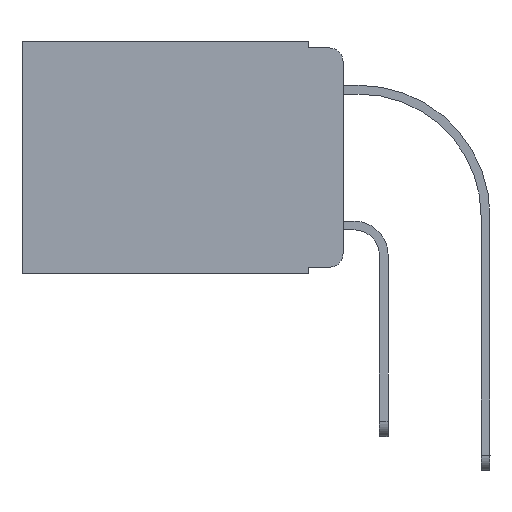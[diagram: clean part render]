
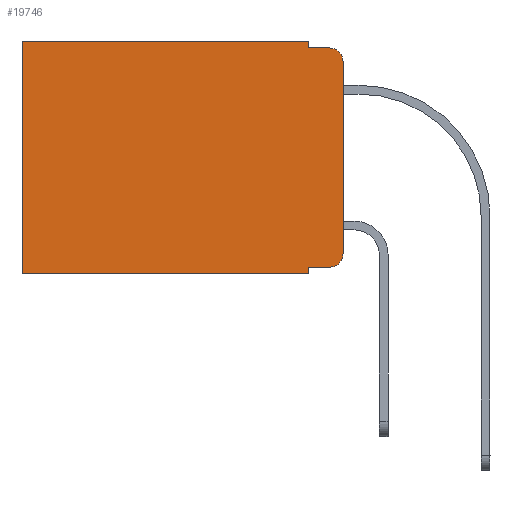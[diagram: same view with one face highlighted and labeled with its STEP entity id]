
A CAD part, left-side view. The second image highlights one B-rep face of the part: STEP entity #19746.
In plain terms, the highlighted planar face has unit normal (-1, 0, 0).
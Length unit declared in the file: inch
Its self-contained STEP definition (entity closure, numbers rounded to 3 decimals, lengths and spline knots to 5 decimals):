
#467 = LINE ( 'NONE', #2227, #14826 ) ;
#669 = CARTESIAN_POINT ( 'NONE',  ( 0.298, 0.051, -0.333 ) ) ;
#692 = DIRECTION ( 'NONE',  ( 0., -1., 0. ) ) ;
#709 = VECTOR ( 'NONE', #11517, 39.37008 ) ;
#900 = CARTESIAN_POINT ( 'NONE',  ( 0.298, 0.473, -0.343 ) ) ;
#1210 = VERTEX_POINT ( 'NONE', #2211 ) ;
#1388 = LINE ( 'NONE', #24292, #19934 ) ;
#1460 = DIRECTION ( 'NONE',  ( -1., 0., 0. ) ) ;
#1543 = CARTESIAN_POINT ( 'NONE',  ( 0.298, 0., 0. ) ) ;
#1808 = ORIENTED_EDGE ( 'NONE', *, *, #18998, .F. ) ;
#1936 = VERTEX_POINT ( 'NONE', #669 ) ;
#2211 = CARTESIAN_POINT ( 'NONE',  ( 0.298, 0.02, -0.01 ) ) ;
#2227 = CARTESIAN_POINT ( 'NONE',  ( 0.298, 0.473, 0. ) ) ;
#2429 = CARTESIAN_POINT ( 'NONE',  ( 0.298, 0.051, -0.01 ) ) ;
#2493 = VECTOR ( 'NONE', #692, 39.37008 ) ;
#3457 = VERTEX_POINT ( 'NONE', #18289 ) ;
#4311 = CIRCLE ( 'NONE', #19516, 0.02 ) ;
#4372 = EDGE_CURVE ( 'NONE', #1936, #24641, #10007, .T. ) ;
#4535 = ORIENTED_EDGE ( 'NONE', *, *, #16667, .F. ) ;
#4623 = ORIENTED_EDGE ( 'NONE', *, *, #20258, .T. ) ;
#4894 = VECTOR ( 'NONE', #12229, 39.37008 ) ;
#5232 = ORIENTED_EDGE ( 'NONE', *, *, #9940, .T. ) ;
#6278 = ORIENTED_EDGE ( 'NONE', *, *, #4372, .T. ) ;
#8195 = PLANE ( 'NONE',  #19969 ) ;
#8224 = CARTESIAN_POINT ( 'NONE',  ( 0.298, 0.051, 0. ) ) ;
#8313 = LINE ( 'NONE', #10929, #18620 ) ;
#8447 = DIRECTION ( 'NONE',  ( 1., 0., 0. ) ) ;
#8999 = VERTEX_POINT ( 'NONE', #2429 ) ;
#9044 = DIRECTION ( 'NONE',  ( 0., 0., -1. ) ) ;
#9327 = DIRECTION ( 'NONE',  ( 0., 1., 0. ) ) ;
#9650 = ORIENTED_EDGE ( 'NONE', *, *, #10064, .F. ) ;
#9698 = ORIENTED_EDGE ( 'NONE', *, *, #10687, .T. ) ;
#9940 = EDGE_CURVE ( 'NONE', #18014, #24470, #467, .T. ) ;
#10007 = LINE ( 'NONE', #19175, #709 ) ;
#10058 = FACE_OUTER_BOUND ( 'NONE', #11805, .T. ) ;
#10064 = EDGE_CURVE ( 'NONE', #17856, #8999, #12722, .T. ) ;
#10212 = CARTESIAN_POINT ( 'NONE',  ( 0.298, 0.051, -0.01 ) ) ;
#10311 = EDGE_CURVE ( 'NONE', #17488, #1210, #13729, .T. ) ;
#10426 = DIRECTION ( 'NONE',  ( 0., 0., -1. ) ) ;
#10448 = LINE ( 'NONE', #10212, #2493 ) ;
#10454 = ORIENTED_EDGE ( 'NONE', *, *, #10311, .T. ) ;
#10687 = EDGE_CURVE ( 'NONE', #17856, #18014, #19092, .T. ) ;
#10929 = CARTESIAN_POINT ( 'NONE',  ( 0.298, 0., -0.343 ) ) ;
#11517 = DIRECTION ( 'NONE',  ( 0., -1., 0. ) ) ;
#11782 = DIRECTION ( 'NONE',  ( 0., 0., -1. ) ) ;
#11805 = EDGE_LOOP ( 'NONE', ( #1808, #10454, #4535, #9650, #9698, #5232, #22938, #22150, #6278, #4623 ) ) ;
#12115 = DIRECTION ( 'NONE',  ( 0., 0., -1. ) ) ;
#12229 = DIRECTION ( 'NONE',  ( 0., 0., -1. ) ) ;
#12579 = CARTESIAN_POINT ( 'NONE',  ( 0.298, 0.473, 0. ) ) ;
#12722 = LINE ( 'NONE', #16510, #17724 ) ;
#12930 = VERTEX_POINT ( 'NONE', #23372 ) ;
#13729 = CIRCLE ( 'NONE', #17336, 0.02 ) ;
#14606 = CARTESIAN_POINT ( 'NONE',  ( 0.298, 0.051, 0. ) ) ;
#14826 = VECTOR ( 'NONE', #12115, 39.37008 ) ;
#14989 = DIRECTION ( 'NONE',  ( 0., 0., -1. ) ) ;
#15837 = CARTESIAN_POINT ( 'NONE',  ( 0.298, 0., 0. ) ) ;
#16268 = CARTESIAN_POINT ( 'NONE',  ( 0.298, 0., -0.03 ) ) ;
#16510 = CARTESIAN_POINT ( 'NONE',  ( 0.298, 0.051, 0. ) ) ;
#16667 = EDGE_CURVE ( 'NONE', #8999, #1210, #10448, .T. ) ;
#17336 = AXIS2_PLACEMENT_3D ( 'NONE', #18635, #1460, #14989 ) ;
#17488 = VERTEX_POINT ( 'NONE', #16268 ) ;
#17724 = VECTOR ( 'NONE', #18376, 39.37008 ) ;
#17856 = VERTEX_POINT ( 'NONE', #8224 ) ;
#18014 = VERTEX_POINT ( 'NONE', #12579 ) ;
#18050 = DIRECTION ( 'NONE',  ( -1., 0., 0. ) ) ;
#18289 = CARTESIAN_POINT ( 'NONE',  ( 0.298, 0.051, -0.343 ) ) ;
#18376 = DIRECTION ( 'NONE',  ( 0., 0., -1. ) ) ;
#18438 = EDGE_CURVE ( 'NONE', #3457, #24470, #8313, .T. ) ;
#18502 = VECTOR ( 'NONE', #9327, 39.37008 ) ;
#18581 = DIRECTION ( 'NONE',  ( 0., 1., 0. ) ) ;
#18620 = VECTOR ( 'NONE', #18581, 39.37008 ) ;
#18635 = CARTESIAN_POINT ( 'NONE',  ( 0.298, 0.02, -0.03 ) ) ;
#18998 = EDGE_CURVE ( 'NONE', #17488, #12930, #1388, .T. ) ;
#19092 = LINE ( 'NONE', #1543, #18502 ) ;
#19175 = CARTESIAN_POINT ( 'NONE',  ( 0.298, 0.051, -0.333 ) ) ;
#19516 = AXIS2_PLACEMENT_3D ( 'NONE', #21554, #18050, #11782 ) ;
#19746 = ADVANCED_FACE ( 'NONE', ( #10058 ), #8195, .F. ) ;
#19854 = CARTESIAN_POINT ( 'NONE',  ( 0.298, 0.02, -0.333 ) ) ;
#19934 = VECTOR ( 'NONE', #9044, 39.37008 ) ;
#19969 = AXIS2_PLACEMENT_3D ( 'NONE', #15837, #8447, #10426 ) ;
#20258 = EDGE_CURVE ( 'NONE', #24641, #12930, #4311, .T. ) ;
#21554 = CARTESIAN_POINT ( 'NONE',  ( 0.298, 0.02, -0.313 ) ) ;
#21755 = LINE ( 'NONE', #14606, #4894 ) ;
#22150 = ORIENTED_EDGE ( 'NONE', *, *, #23533, .F. ) ;
#22938 = ORIENTED_EDGE ( 'NONE', *, *, #18438, .F. ) ;
#23372 = CARTESIAN_POINT ( 'NONE',  ( 0.298, 0., -0.313 ) ) ;
#23533 = EDGE_CURVE ( 'NONE', #1936, #3457, #21755, .T. ) ;
#24292 = CARTESIAN_POINT ( 'NONE',  ( 0.298, 0., 0. ) ) ;
#24470 = VERTEX_POINT ( 'NONE', #900 ) ;
#24641 = VERTEX_POINT ( 'NONE', #19854 ) ;
